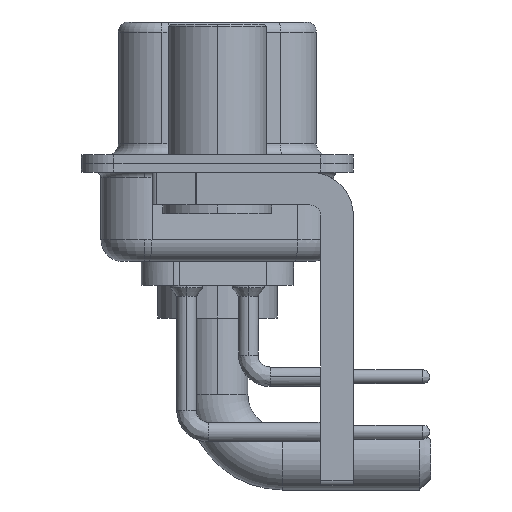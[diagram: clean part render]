
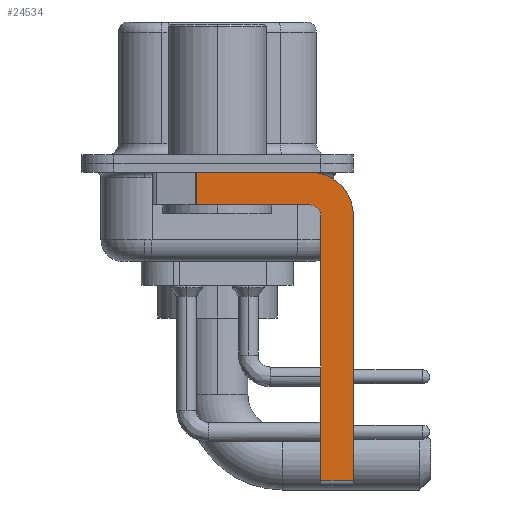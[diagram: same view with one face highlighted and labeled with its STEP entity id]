
A CAD part, left-side view. The second image highlights one B-rep face of the part: STEP entity #24534.
In plain terms, the highlighted planar face has unit normal (-1, 0, 0).
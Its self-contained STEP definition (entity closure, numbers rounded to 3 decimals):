
#22 = CARTESIAN_POINT ( 'NONE',  ( -2.9, -4.25, -1.9 ) ) ;
#838 = VERTEX_POINT ( 'NONE', #20282 ) ;
#1133 = VERTEX_POINT ( 'NONE', #12284 ) ;
#1174 = VECTOR ( 'NONE', #12720, 1000. ) ;
#1363 = EDGE_CURVE ( 'NONE', #3889, #22261, #9004, .T. ) ;
#1434 = EDGE_CURVE ( 'NONE', #3889, #1133, #24354, .T. ) ;
#1466 = VERTEX_POINT ( 'NONE', #5842 ) ;
#1541 = DIRECTION ( 'NONE',  ( 0., 0., -1. ) ) ;
#1696 = CARTESIAN_POINT ( 'NONE',  ( -2.9, 3., -0.4 ) ) ;
#2371 = DIRECTION ( 'NONE',  ( 0., 0., 1. ) ) ;
#2384 = VECTOR ( 'NONE', #11240, 1000. ) ;
#2746 = CARTESIAN_POINT ( 'NONE',  ( -2.9, -6.25, -2.4 ) ) ;
#2869 = CARTESIAN_POINT ( 'NONE',  ( -2.9, -4.25, -1.9 ) ) ;
#3889 = VERTEX_POINT ( 'NONE', #7249 ) ;
#3926 = CARTESIAN_POINT ( 'NONE',  ( -2.9, -6.25, -2.4 ) ) ;
#5049 = LINE ( 'NONE', #24181, #1174 ) ;
#5527 = CIRCLE ( 'NONE', #19613, 2. ) ;
#5842 = CARTESIAN_POINT ( 'NONE',  ( -2.9, -6.25, -14.55 ) ) ;
#6650 = DIRECTION ( 'NONE',  ( 0., 0., -1. ) ) ;
#6914 = VECTOR ( 'NONE', #17511, 1000. ) ;
#7113 = CARTESIAN_POINT ( 'NONE',  ( -2.9, 0.978, -1.9 ) ) ;
#7249 = CARTESIAN_POINT ( 'NONE',  ( -2.9, 0.978, -0.4 ) ) ;
#7307 = EDGE_CURVE ( 'NONE', #1133, #21028, #5527, .T. ) ;
#7340 = CARTESIAN_POINT ( 'NONE',  ( -2.9, -4.75, -14.8 ) ) ;
#7350 = ORIENTED_EDGE ( 'NONE', *, *, #12781, .F. ) ;
#7657 = EDGE_CURVE ( 'NONE', #838, #12947, #24053, .T. ) ;
#7971 = AXIS2_PLACEMENT_3D ( 'NONE', #12045, #11919, #2371 ) ;
#8515 = EDGE_CURVE ( 'NONE', #8527, #838, #15263, .T. ) ;
#8527 = VERTEX_POINT ( 'NONE', #15140 ) ;
#8578 = ORIENTED_EDGE ( 'NONE', *, *, #8750, .T. ) ;
#8750 = EDGE_CURVE ( 'NONE', #8527, #1466, #5049, .T. ) ;
#8794 = FACE_OUTER_BOUND ( 'NONE', #15035, .T. ) ;
#9004 = LINE ( 'NONE', #7113, #23990 ) ;
#11240 = DIRECTION ( 'NONE',  ( 0., 0., 1. ) ) ;
#11470 = LINE ( 'NONE', #3926, #15793 ) ;
#11908 = AXIS2_PLACEMENT_3D ( 'NONE', #23901, #24144, #6650 ) ;
#11919 = DIRECTION ( 'NONE',  ( -1., 0., 0. ) ) ;
#12045 = CARTESIAN_POINT ( 'NONE',  ( -2.9, -4.25, -2.4 ) ) ;
#12284 = CARTESIAN_POINT ( 'NONE',  ( -2.9, -4.25, -0.4 ) ) ;
#12606 = CARTESIAN_POINT ( 'NONE',  ( -2.9, 0.978, -1.9 ) ) ;
#12720 = DIRECTION ( 'NONE',  ( 0., -1., 0. ) ) ;
#12781 = EDGE_CURVE ( 'NONE', #21028, #1466, #11470, .T. ) ;
#12837 = ORIENTED_EDGE ( 'NONE', *, *, #7307, .F. ) ;
#12947 = VERTEX_POINT ( 'NONE', #2869 ) ;
#13219 = ORIENTED_EDGE ( 'NONE', *, *, #8515, .F. ) ;
#13710 = CARTESIAN_POINT ( 'NONE',  ( -2.9, -4.25, -2.4 ) ) ;
#13974 = DIRECTION ( 'NONE',  ( 1., 0., 0. ) ) ;
#14761 = ORIENTED_EDGE ( 'NONE', *, *, #18251, .F. ) ;
#14792 = DIRECTION ( 'NONE',  ( 0., 0., -1. ) ) ;
#15035 = EDGE_LOOP ( 'NONE', ( #21731, #22966, #14761, #23760, #13219, #8578, #7350, #12837 ) ) ;
#15140 = CARTESIAN_POINT ( 'NONE',  ( -2.9, -4.75, -14.55 ) ) ;
#15263 = LINE ( 'NONE', #7340, #2384 ) ;
#15522 = VECTOR ( 'NONE', #16809, 1000. ) ;
#15716 = DIRECTION ( 'NONE',  ( 0., 0., -1. ) ) ;
#15793 = VECTOR ( 'NONE', #1541, 1000. ) ;
#16208 = PLANE ( 'NONE',  #11908 ) ;
#16809 = DIRECTION ( 'NONE',  ( 0., -1., 0. ) ) ;
#17511 = DIRECTION ( 'NONE',  ( 0., 1., 0. ) ) ;
#18251 = EDGE_CURVE ( 'NONE', #12947, #22261, #22556, .T. ) ;
#19613 = AXIS2_PLACEMENT_3D ( 'NONE', #13710, #13974, #15716 ) ;
#20282 = CARTESIAN_POINT ( 'NONE',  ( -2.9, -4.75, -2.4 ) ) ;
#21028 = VERTEX_POINT ( 'NONE', #2746 ) ;
#21731 = ORIENTED_EDGE ( 'NONE', *, *, #1434, .F. ) ;
#22261 = VERTEX_POINT ( 'NONE', #12606 ) ;
#22556 = LINE ( 'NONE', #22, #6914 ) ;
#22966 = ORIENTED_EDGE ( 'NONE', *, *, #1363, .T. ) ;
#23760 = ORIENTED_EDGE ( 'NONE', *, *, #7657, .F. ) ;
#23901 = CARTESIAN_POINT ( 'NONE',  ( -2.9, -4.25, -2.4 ) ) ;
#23990 = VECTOR ( 'NONE', #14792, 1000. ) ;
#24053 = CIRCLE ( 'NONE', #7971, 0.5 ) ;
#24144 = DIRECTION ( 'NONE',  ( 1., 0., 0. ) ) ;
#24181 = CARTESIAN_POINT ( 'NONE',  ( -2.9, -4.25, -14.55 ) ) ;
#24354 = LINE ( 'NONE', #1696, #15522 ) ;
#24534 = ADVANCED_FACE ( 'NONE', ( #8794 ), #16208, .F. ) ;
